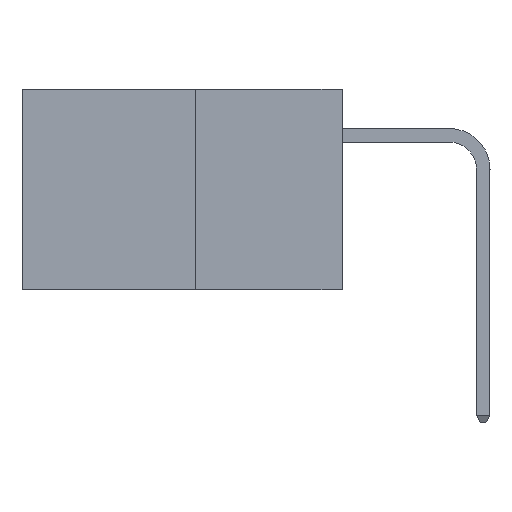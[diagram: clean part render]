
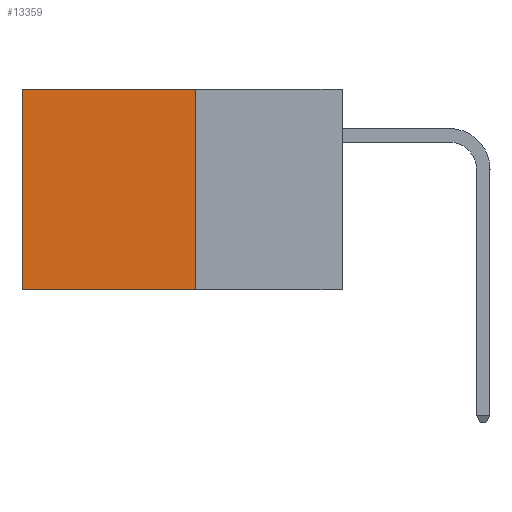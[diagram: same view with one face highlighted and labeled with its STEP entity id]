
A CAD part, left-side view. The second image highlights one B-rep face of the part: STEP entity #13359.
In plain terms, the highlighted planar face has unit normal (-1, 0, 0).
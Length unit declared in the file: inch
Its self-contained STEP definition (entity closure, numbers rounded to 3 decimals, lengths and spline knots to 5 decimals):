
#150 = EDGE_CURVE ( 'NONE', #22455, #910, #17483, .T. ) ;
#910 = VERTEX_POINT ( 'NONE', #3864 ) ;
#2224 = VECTOR ( 'NONE', #9156, 39.37008 ) ;
#2284 = LINE ( 'NONE', #7701, #12933 ) ;
#3702 = PLANE ( 'NONE',  #7719 ) ;
#3710 = VERTEX_POINT ( 'NONE', #4375 ) ;
#3864 = CARTESIAN_POINT ( 'NONE',  ( 0.277, 0.27, -0.37 ) ) ;
#4375 = CARTESIAN_POINT ( 'NONE',  ( 0.277, 0.59, -0.37 ) ) ;
#6815 = ORIENTED_EDGE ( 'NONE', *, *, #18920, .F. ) ;
#7066 = CARTESIAN_POINT ( 'NONE',  ( 0.277, 0.27, 0. ) ) ;
#7405 = CARTESIAN_POINT ( 'NONE',  ( 0.277, 0.27, -0.37 ) ) ;
#7475 = DIRECTION ( 'NONE',  ( 0., 0., -1. ) ) ;
#7701 = CARTESIAN_POINT ( 'NONE',  ( 0.277, 0.27, -0.37 ) ) ;
#7719 = AXIS2_PLACEMENT_3D ( 'NONE', #17687, #19686, #7761 ) ;
#7761 = DIRECTION ( 'NONE',  ( 0., 0., -1. ) ) ;
#8769 = EDGE_CURVE ( 'NONE', #22455, #19059, #12870, .T. ) ;
#9156 = DIRECTION ( 'NONE',  ( 0., 1., 0. ) ) ;
#9819 = ORIENTED_EDGE ( 'NONE', *, *, #21666, .T. ) ;
#11501 = DIRECTION ( 'NONE',  ( 0., 0., -1. ) ) ;
#12870 = LINE ( 'NONE', #7066, #2224 ) ;
#12933 = VECTOR ( 'NONE', #21633, 39.37008 ) ;
#13359 = ADVANCED_FACE ( 'NONE', ( #19781 ), #3702, .F. ) ;
#14816 = ORIENTED_EDGE ( 'NONE', *, *, #150, .F. ) ;
#15425 = CARTESIAN_POINT ( 'NONE',  ( 0.277, 0.59, -0.37 ) ) ;
#17483 = LINE ( 'NONE', #7405, #18111 ) ;
#17687 = CARTESIAN_POINT ( 'NONE',  ( 0.277, 0.27, -0.37 ) ) ;
#18060 = CARTESIAN_POINT ( 'NONE',  ( 0.277, 0.59, 0. ) ) ;
#18111 = VECTOR ( 'NONE', #7475, 39.37008 ) ;
#18877 = VECTOR ( 'NONE', #11501, 39.37008 ) ;
#18920 = EDGE_CURVE ( 'NONE', #910, #3710, #2284, .T. ) ;
#19059 = VERTEX_POINT ( 'NONE', #18060 ) ;
#19686 = DIRECTION ( 'NONE',  ( 1., 0., 0. ) ) ;
#19781 = FACE_OUTER_BOUND ( 'NONE', #24888, .T. ) ;
#21633 = DIRECTION ( 'NONE',  ( 0., 1., 0. ) ) ;
#21666 = EDGE_CURVE ( 'NONE', #19059, #3710, #24172, .T. ) ;
#22170 = CARTESIAN_POINT ( 'NONE',  ( 0.277, 0.27, 0. ) ) ;
#22455 = VERTEX_POINT ( 'NONE', #22170 ) ;
#23352 = ORIENTED_EDGE ( 'NONE', *, *, #8769, .T. ) ;
#24172 = LINE ( 'NONE', #15425, #18877 ) ;
#24888 = EDGE_LOOP ( 'NONE', ( #9819, #6815, #14816, #23352 ) ) ;
